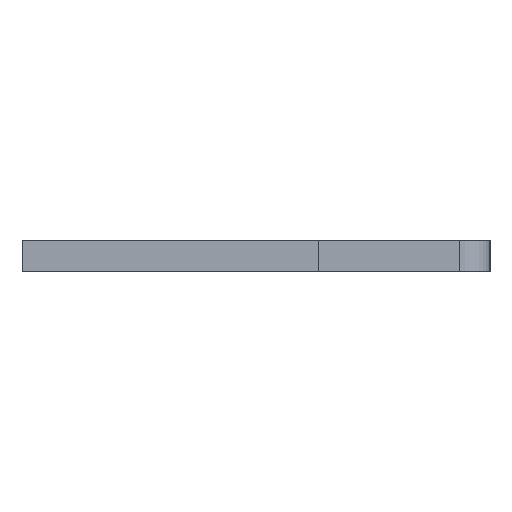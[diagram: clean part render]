
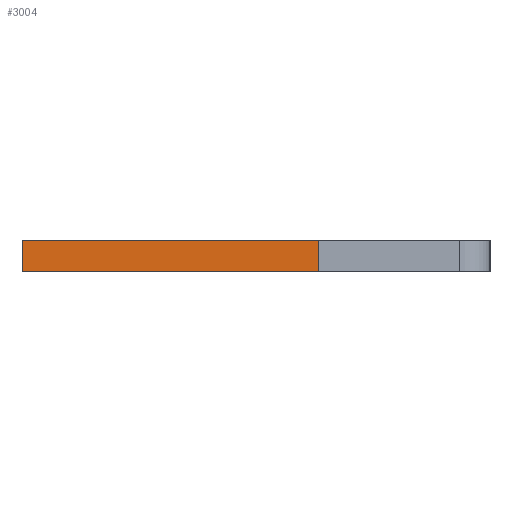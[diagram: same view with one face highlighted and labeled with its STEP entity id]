
A CAD part, left-side view. The second image highlights one B-rep face of the part: STEP entity #3004.
In plain terms, the highlighted face is planar.
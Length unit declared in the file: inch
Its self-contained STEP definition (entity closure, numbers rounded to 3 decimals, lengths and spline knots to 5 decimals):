
#20 = CARTESIAN_POINT ( 'NONE',  ( 0.01, 0.15, -0.04 ) ) ;
#171 = VERTEX_POINT ( 'NONE', #664 ) ;
#192 = PLANE ( 'NONE',  #1837 ) ;
#235 = LINE ( 'NONE', #2271, #1803 ) ;
#371 = DIRECTION ( 'NONE',  ( 0., 1., 0. ) ) ;
#413 = CARTESIAN_POINT ( 'NONE',  ( 0.01, -0.04, -0.04 ) ) ;
#513 = VECTOR ( 'NONE', #565, 39.37008 ) ;
#565 = DIRECTION ( 'NONE',  ( 0., 1., 0. ) ) ;
#664 = CARTESIAN_POINT ( 'NONE',  ( 0.01, 0.15, -0.04 ) ) ;
#719 = DIRECTION ( 'NONE',  ( -1., 0., 0. ) ) ;
#788 = VERTEX_POINT ( 'NONE', #1862 ) ;
#856 = EDGE_CURVE ( 'NONE', #171, #2670, #1652, .T. ) ;
#1276 = ORIENTED_EDGE ( 'NONE', *, *, #1913, .F. ) ;
#1339 = CARTESIAN_POINT ( 'NONE',  ( -0.01, -0.04, -0.04 ) ) ;
#1347 = CARTESIAN_POINT ( 'NONE',  ( -0.01, 0.15, -0.04 ) ) ;
#1451 = DIRECTION ( 'NONE',  ( 0., 0., 1. ) ) ;
#1579 = CARTESIAN_POINT ( 'NONE',  ( 0.01, 0.15, -0.04 ) ) ;
#1614 = ORIENTED_EDGE ( 'NONE', *, *, #2432, .T. ) ;
#1652 = LINE ( 'NONE', #20, #1696 ) ;
#1696 = VECTOR ( 'NONE', #719, 39.37008 ) ;
#1734 = ORIENTED_EDGE ( 'NONE', *, *, #1830, .T. ) ;
#1796 = FACE_OUTER_BOUND ( 'NONE', #1999, .T. ) ;
#1803 = VECTOR ( 'NONE', #371, 39.37008 ) ;
#1826 = DIRECTION ( 'NONE',  ( -1., 0., 0. ) ) ;
#1830 = EDGE_CURVE ( 'NONE', #2936, #2670, #235, .T. ) ;
#1837 = AXIS2_PLACEMENT_3D ( 'NONE', #1579, #1451, #2379 ) ;
#1862 = CARTESIAN_POINT ( 'NONE',  ( 0.01, -0.04, -0.04 ) ) ;
#1913 = EDGE_CURVE ( 'NONE', #788, #171, #2622, .T. ) ;
#1999 = EDGE_LOOP ( 'NONE', ( #1734, #2740, #1276, #1614 ) ) ;
#2271 = CARTESIAN_POINT ( 'NONE',  ( -0.01, 0.15, -0.04 ) ) ;
#2379 = DIRECTION ( 'NONE',  ( 1., 0., 0. ) ) ;
#2412 = CARTESIAN_POINT ( 'NONE',  ( 0.01, 0.15, -0.04 ) ) ;
#2432 = EDGE_CURVE ( 'NONE', #788, #2936, #2556, .T. ) ;
#2556 = LINE ( 'NONE', #413, #2735 ) ;
#2622 = LINE ( 'NONE', #2412, #513 ) ;
#2670 = VERTEX_POINT ( 'NONE', #1347 ) ;
#2735 = VECTOR ( 'NONE', #1826, 39.37008 ) ;
#2740 = ORIENTED_EDGE ( 'NONE', *, *, #856, .F. ) ;
#2936 = VERTEX_POINT ( 'NONE', #1339 ) ;
#3004 = ADVANCED_FACE ( 'NONE', ( #1796 ), #192, .F. ) ;
